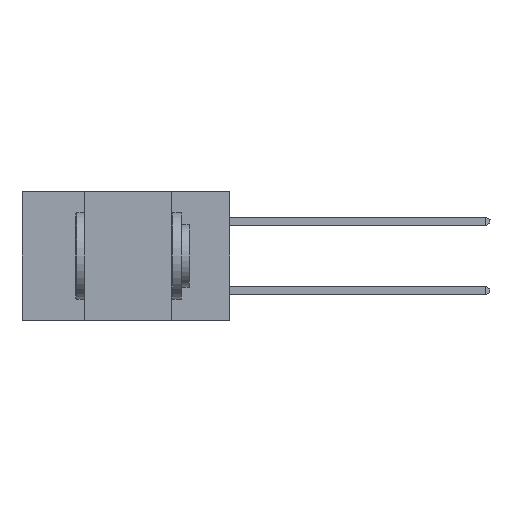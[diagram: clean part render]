
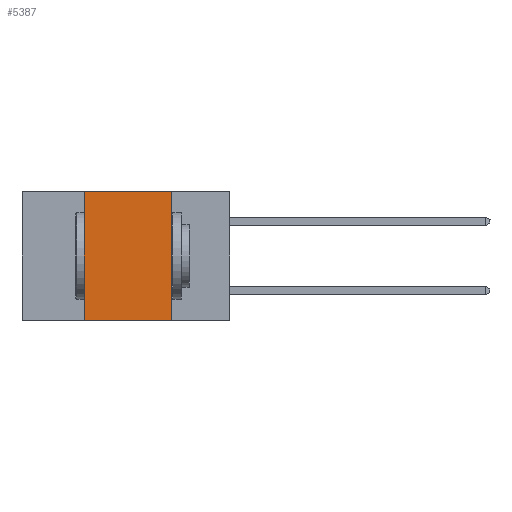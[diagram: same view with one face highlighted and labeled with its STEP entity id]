
A CAD part, left-side view. The second image highlights one B-rep face of the part: STEP entity #5387.
In plain terms, the highlighted planar face has unit normal (-1, 0, 0).
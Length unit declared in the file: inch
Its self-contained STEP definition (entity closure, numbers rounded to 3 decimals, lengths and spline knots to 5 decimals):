
#3070 = AXIS2_PLACEMENT_3D ( 'NONE', #14728, #19518, #5507 ) ;
#3674 = VECTOR ( 'NONE', #19804, 39.37008 ) ;
#3949 = ORIENTED_EDGE ( 'NONE', *, *, #18179, .F. ) ;
#3956 = DIRECTION ( 'NONE',  ( 0., -1., 0. ) ) ;
#3975 = CARTESIAN_POINT ( 'NONE',  ( 0., 0.42, -0.37 ) ) ;
#4181 = CARTESIAN_POINT ( 'NONE',  ( 0., 0.6, -0.37 ) ) ;
#4191 = CARTESIAN_POINT ( 'NONE',  ( 0., 0.42, 0. ) ) ;
#5050 = VECTOR ( 'NONE', #3956, 39.37008 ) ;
#5193 = ORIENTED_EDGE ( 'NONE', *, *, #20366, .F. ) ;
#5196 = PLANE ( 'NONE',  #3070 ) ;
#5387 = ADVANCED_FACE ( 'NONE', ( #13050 ), #5196, .F. ) ;
#5507 = DIRECTION ( 'NONE',  ( 0., 0., -1. ) ) ;
#7200 = CARTESIAN_POINT ( 'NONE',  ( 0., 0.6, 0. ) ) ;
#7324 = VECTOR ( 'NONE', #12360, 39.37008 ) ;
#8630 = ORIENTED_EDGE ( 'NONE', *, *, #18931, .F. ) ;
#8733 = CARTESIAN_POINT ( 'NONE',  ( 0., 0.17, -0.37 ) ) ;
#9337 = VERTEX_POINT ( 'NONE', #4191 ) ;
#10192 = ORIENTED_EDGE ( 'NONE', *, *, #18113, .T. ) ;
#12211 = VERTEX_POINT ( 'NONE', #13499 ) ;
#12253 = DIRECTION ( 'NONE',  ( 0., -1., 0. ) ) ;
#12360 = DIRECTION ( 'NONE',  ( 0., 0., 1. ) ) ;
#13050 = FACE_OUTER_BOUND ( 'NONE', #20160, .T. ) ;
#13398 = CARTESIAN_POINT ( 'NONE',  ( 0., 0.42, -0.37 ) ) ;
#13499 = CARTESIAN_POINT ( 'NONE',  ( 0., 0.17, 0. ) ) ;
#13541 = CARTESIAN_POINT ( 'NONE',  ( 0., 0.17, -0.37 ) ) ;
#13685 = VECTOR ( 'NONE', #12253, 39.37008 ) ;
#14728 = CARTESIAN_POINT ( 'NONE',  ( 0., 0.6, 0. ) ) ;
#15484 = LINE ( 'NONE', #3975, #7324 ) ;
#16264 = VERTEX_POINT ( 'NONE', #13541 ) ;
#16780 = LINE ( 'NONE', #8733, #3674 ) ;
#18113 = EDGE_CURVE ( 'NONE', #19846, #16264, #18604, .T. ) ;
#18179 = EDGE_CURVE ( 'NONE', #19846, #9337, #15484, .T. ) ;
#18585 = LINE ( 'NONE', #7200, #5050 ) ;
#18604 = LINE ( 'NONE', #4181, #13685 ) ;
#18931 = EDGE_CURVE ( 'NONE', #12211, #16264, #16780, .T. ) ;
#19518 = DIRECTION ( 'NONE',  ( 1., 0., 0. ) ) ;
#19804 = DIRECTION ( 'NONE',  ( 0., 0., -1. ) ) ;
#19846 = VERTEX_POINT ( 'NONE', #13398 ) ;
#20160 = EDGE_LOOP ( 'NONE', ( #8630, #5193, #3949, #10192 ) ) ;
#20366 = EDGE_CURVE ( 'NONE', #9337, #12211, #18585, .T. ) ;
